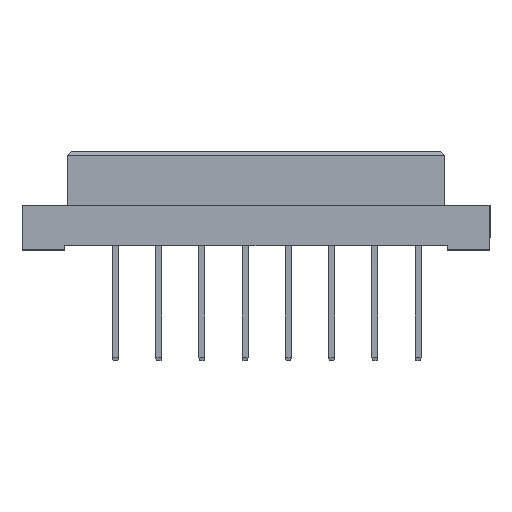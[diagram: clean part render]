
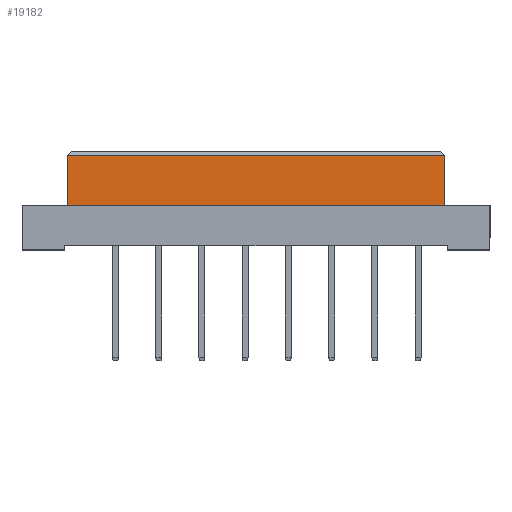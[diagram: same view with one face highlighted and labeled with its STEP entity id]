
A CAD part, top view. The second image highlights one B-rep face of the part: STEP entity #19182.
In plain terms, the highlighted planar face has unit normal (0, 0, 1).
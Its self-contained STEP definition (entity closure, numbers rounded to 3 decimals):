
#51 = LINE ( 'NONE', #18853, #18993 ) ;
#403 = FACE_OUTER_BOUND ( 'NONE', #4797, .T. ) ;
#780 = LINE ( 'NONE', #16888, #7741 ) ;
#1005 = LINE ( 'NONE', #5890, #19739 ) ;
#2094 = CARTESIAN_POINT ( 'NONE',  ( -22.2, -6.4, 4.25 ) ) ;
#4457 = CARTESIAN_POINT ( 'NONE',  ( -22.2, -0.5, 4.25 ) ) ;
#4797 = EDGE_LOOP ( 'NONE', ( #13069, #13433, #19741, #16898 ) ) ;
#4805 = DIRECTION ( 'NONE',  ( -1., 0., 0. ) ) ;
#5455 = VECTOR ( 'NONE', #11834, 1000. ) ;
#5479 = LINE ( 'NONE', #8375, #5455 ) ;
#5890 = CARTESIAN_POINT ( 'NONE',  ( 22.2, -6.4, 4.25 ) ) ;
#7361 = VERTEX_POINT ( 'NONE', #4457 ) ;
#7741 = VECTOR ( 'NONE', #16473, 1000. ) ;
#8112 = EDGE_CURVE ( 'NONE', #8450, #7361, #780, .T. ) ;
#8288 = DIRECTION ( 'NONE',  ( 0., 0., 1. ) ) ;
#8375 = CARTESIAN_POINT ( 'NONE',  ( 22.2, -6.4, 4.25 ) ) ;
#8434 = CARTESIAN_POINT ( 'NONE',  ( 22.2, -0.5, 4.25 ) ) ;
#8450 = VERTEX_POINT ( 'NONE', #2094 ) ;
#8501 = PLANE ( 'NONE',  #20281 ) ;
#11121 = EDGE_CURVE ( 'NONE', #8450, #12881, #5479, .T. ) ;
#11270 = EDGE_CURVE ( 'NONE', #12881, #16027, #1005, .T. ) ;
#11777 = EDGE_CURVE ( 'NONE', #16027, #7361, #51, .T. ) ;
#11834 = DIRECTION ( 'NONE',  ( 1., 0., 0. ) ) ;
#12249 = DIRECTION ( 'NONE',  ( 0., 1., 0. ) ) ;
#12881 = VERTEX_POINT ( 'NONE', #19068 ) ;
#13069 = ORIENTED_EDGE ( 'NONE', *, *, #11270, .T. ) ;
#13433 = ORIENTED_EDGE ( 'NONE', *, *, #11777, .T. ) ;
#16027 = VERTEX_POINT ( 'NONE', #8434 ) ;
#16473 = DIRECTION ( 'NONE',  ( 0., 1., 0. ) ) ;
#16888 = CARTESIAN_POINT ( 'NONE',  ( -22.2, -6.4, 4.25 ) ) ;
#16898 = ORIENTED_EDGE ( 'NONE', *, *, #11121, .T. ) ;
#17849 = DIRECTION ( 'NONE',  ( 1., 0., 0. ) ) ;
#18853 = CARTESIAN_POINT ( 'NONE',  ( -22.2, -0.5, 4.25 ) ) ;
#18993 = VECTOR ( 'NONE', #4805, 1000. ) ;
#19068 = CARTESIAN_POINT ( 'NONE',  ( 22.2, -6.4, 4.25 ) ) ;
#19182 = ADVANCED_FACE ( 'NONE', ( #403 ), #8501, .T. ) ;
#19739 = VECTOR ( 'NONE', #12249, 1000. ) ;
#19741 = ORIENTED_EDGE ( 'NONE', *, *, #8112, .F. ) ;
#19747 = CARTESIAN_POINT ( 'NONE',  ( 22.2, -6.4, 4.25 ) ) ;
#20281 = AXIS2_PLACEMENT_3D ( 'NONE', #19747, #8288, #17849 ) ;
